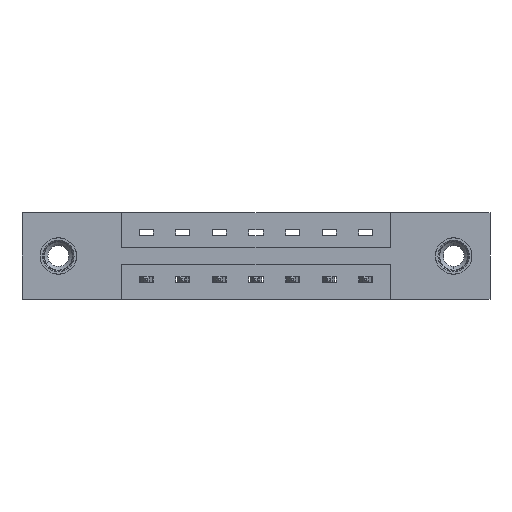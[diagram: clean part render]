
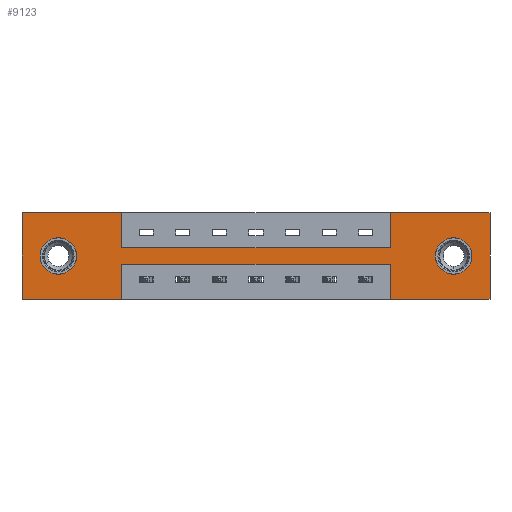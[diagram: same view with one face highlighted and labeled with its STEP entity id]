
A CAD part, front view. The second image highlights one B-rep face of the part: STEP entity #9123.
In plain terms, the highlighted planar face has unit normal (0, -1, 0).
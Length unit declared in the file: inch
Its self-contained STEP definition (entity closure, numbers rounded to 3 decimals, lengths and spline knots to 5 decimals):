
#80 = CIRCLE ( 'NONE', #4059, 0.078 ) ;
#174 = CARTESIAN_POINT ( 'NONE',  ( 1.573, 0., 0. ) ) ;
#193 = ORIENTED_EDGE ( 'NONE', *, *, #5267, .F. ) ;
#200 = DIRECTION ( 'NONE',  ( 0., 0., 1. ) ) ;
#205 = EDGE_CURVE ( 'NONE', #1161, #3313, #1393, .T. ) ;
#228 = VERTEX_POINT ( 'NONE', #9288 ) ;
#248 = DIRECTION ( 'NONE',  ( 0., 0., -1. ) ) ;
#309 = DIRECTION ( 'NONE',  ( 0., 0., -1. ) ) ;
#322 = VERTEX_POINT ( 'NONE', #9182 ) ;
#593 = EDGE_LOOP ( 'NONE', ( #8282, #1849 ) ) ;
#752 = LINE ( 'NONE', #2035, #3151 ) ;
#777 = LINE ( 'NONE', #8391, #4910 ) ;
#796 = LINE ( 'NONE', #4745, #3440 ) ;
#906 = EDGE_CURVE ( 'NONE', #228, #8220, #6104, .T. ) ;
#951 = VERTEX_POINT ( 'NONE', #7539 ) ;
#952 = CARTESIAN_POINT ( 'NONE',  ( 0.155, 0., -0.107 ) ) ;
#957 = ORIENTED_EDGE ( 'NONE', *, *, #2011, .T. ) ;
#1055 = VERTEX_POINT ( 'NONE', #5744 ) ;
#1113 = ORIENTED_EDGE ( 'NONE', *, *, #5197, .F. ) ;
#1161 = VERTEX_POINT ( 'NONE', #8983 ) ;
#1162 = DIRECTION ( 'NONE',  ( 0., 0., 1. ) ) ;
#1353 = FACE_BOUND ( 'NONE', #4217, .T. ) ;
#1393 = CIRCLE ( 'NONE', #2900, 0.078 ) ;
#1439 = CARTESIAN_POINT ( 'NONE',  ( 0.425, 0., -0.15 ) ) ;
#1481 = ORIENTED_EDGE ( 'NONE', *, *, #8433, .F. ) ;
#1596 = EDGE_LOOP ( 'NONE', ( #5784, #8561, #7151, #1766, #6206, #3369, #1481, #5132, #1113, #7271, #3338, #193 ) ) ;
#1640 = CARTESIAN_POINT ( 'NONE',  ( 0.155, 0., -0.185 ) ) ;
#1647 = VECTOR ( 'NONE', #5530, 39.37008 ) ;
#1674 = CARTESIAN_POINT ( 'NONE',  ( 0.155, 0., -0.263 ) ) ;
#1714 = EDGE_CURVE ( 'NONE', #951, #1791, #3684, .T. ) ;
#1766 = ORIENTED_EDGE ( 'NONE', *, *, #8776, .F. ) ;
#1791 = VERTEX_POINT ( 'NONE', #10866 ) ;
#1849 = ORIENTED_EDGE ( 'NONE', *, *, #7267, .T. ) ;
#2001 = VERTEX_POINT ( 'NONE', #952 ) ;
#2011 = EDGE_CURVE ( 'NONE', #10608, #2001, #5579, .T. ) ;
#2035 = CARTESIAN_POINT ( 'NONE',  ( 0., 0., 0. ) ) ;
#2158 = EDGE_CURVE ( 'NONE', #1055, #228, #3672, .T. ) ;
#2446 = CARTESIAN_POINT ( 'NONE',  ( 1.843, 0., -0.185 ) ) ;
#2522 = DIRECTION ( 'NONE',  ( -1., 0., 0. ) ) ;
#2534 = DIRECTION ( 'NONE',  ( 0., 0., 1. ) ) ;
#2651 = ORIENTED_EDGE ( 'NONE', *, *, #6670, .T. ) ;
#2759 = AXIS2_PLACEMENT_3D ( 'NONE', #10273, #5220, #1162 ) ;
#2883 = CARTESIAN_POINT ( 'NONE',  ( 0., 0., 0. ) ) ;
#2900 = AXIS2_PLACEMENT_3D ( 'NONE', #2446, #5797, #4628 ) ;
#3151 = VECTOR ( 'NONE', #200, 39.37008 ) ;
#3251 = LINE ( 'NONE', #3415, #5261 ) ;
#3313 = VERTEX_POINT ( 'NONE', #8738 ) ;
#3338 = ORIENTED_EDGE ( 'NONE', *, *, #10277, .F. ) ;
#3369 = ORIENTED_EDGE ( 'NONE', *, *, #2158, .F. ) ;
#3415 = CARTESIAN_POINT ( 'NONE',  ( 1.573, 0., -0.37 ) ) ;
#3416 = VECTOR ( 'NONE', #7264, 39.37008 ) ;
#3440 = VECTOR ( 'NONE', #309, 39.37008 ) ;
#3475 = CARTESIAN_POINT ( 'NONE',  ( 1.573, 0., -0.37 ) ) ;
#3672 = LINE ( 'NONE', #7025, #1647 ) ;
#3680 = FACE_OUTER_BOUND ( 'NONE', #1596, .T. ) ;
#3684 = LINE ( 'NONE', #2883, #3416 ) ;
#3840 = VECTOR ( 'NONE', #248, 39.37008 ) ;
#3854 = DIRECTION ( 'NONE',  ( -1., 0., 0. ) ) ;
#3856 = DIRECTION ( 'NONE',  ( 0., -1., 0. ) ) ;
#3902 = CARTESIAN_POINT ( 'NONE',  ( 1.998, 0., 0. ) ) ;
#3952 = DIRECTION ( 'NONE',  ( 0., 1., 0. ) ) ;
#4059 = AXIS2_PLACEMENT_3D ( 'NONE', #1640, #7599, #2534 ) ;
#4068 = LINE ( 'NONE', #7775, #8249 ) ;
#4153 = VERTEX_POINT ( 'NONE', #5677 ) ;
#4165 = LINE ( 'NONE', #174, #10171 ) ;
#4217 = EDGE_LOOP ( 'NONE', ( #2651, #957 ) ) ;
#4421 = EDGE_CURVE ( 'NONE', #5087, #10705, #3251, .T. ) ;
#4628 = DIRECTION ( 'NONE',  ( 0., 0., -1. ) ) ;
#4667 = CARTESIAN_POINT ( 'NONE',  ( 0.425, 0., 0. ) ) ;
#4676 = VERTEX_POINT ( 'NONE', #8818 ) ;
#4739 = CARTESIAN_POINT ( 'NONE',  ( 0., 0., -0.37 ) ) ;
#4745 = CARTESIAN_POINT ( 'NONE',  ( 0.425, 0., -0.37 ) ) ;
#4910 = VECTOR ( 'NONE', #2522, 39.37008 ) ;
#5087 = VERTEX_POINT ( 'NONE', #3475 ) ;
#5132 = ORIENTED_EDGE ( 'NONE', *, *, #10719, .F. ) ;
#5197 = EDGE_CURVE ( 'NONE', #1791, #9813, #10594, .T. ) ;
#5220 = DIRECTION ( 'NONE',  ( 0., 1., 0. ) ) ;
#5261 = VECTOR ( 'NONE', #10843, 39.37008 ) ;
#5267 = EDGE_CURVE ( 'NONE', #322, #9967, #7719, .T. ) ;
#5511 = VECTOR ( 'NONE', #3854, 39.37008 ) ;
#5514 = DIRECTION ( 'NONE',  ( 0., 0., -1. ) ) ;
#5530 = DIRECTION ( 'NONE',  ( 1., 0., 0. ) ) ;
#5579 = CIRCLE ( 'NONE', #2759, 0.078 ) ;
#5677 = CARTESIAN_POINT ( 'NONE',  ( 0.425, 0., -0.22 ) ) ;
#5744 = CARTESIAN_POINT ( 'NONE',  ( 1.573, 0., 0. ) ) ;
#5784 = ORIENTED_EDGE ( 'NONE', *, *, #7891, .F. ) ;
#5797 = DIRECTION ( 'NONE',  ( 0., 1., 0. ) ) ;
#5914 = AXIS2_PLACEMENT_3D ( 'NONE', #8937, #3952, #9744 ) ;
#5929 = CARTESIAN_POINT ( 'NONE',  ( 0., 0., -0.37 ) ) ;
#6104 = LINE ( 'NONE', #3902, #3840 ) ;
#6206 = ORIENTED_EDGE ( 'NONE', *, *, #906, .F. ) ;
#6310 = DIRECTION ( 'NONE',  ( 0., 0., 1. ) ) ;
#6670 = EDGE_CURVE ( 'NONE', #2001, #10608, #80, .T. ) ;
#7025 = CARTESIAN_POINT ( 'NONE',  ( 0., 0., 0. ) ) ;
#7151 = ORIENTED_EDGE ( 'NONE', *, *, #4421, .F. ) ;
#7264 = DIRECTION ( 'NONE',  ( 1., 0., 0. ) ) ;
#7267 = EDGE_CURVE ( 'NONE', #3313, #1161, #7561, .T. ) ;
#7271 = ORIENTED_EDGE ( 'NONE', *, *, #1714, .F. ) ;
#7539 = CARTESIAN_POINT ( 'NONE',  ( 0., 0., 0. ) ) ;
#7561 = CIRCLE ( 'NONE', #5914, 0.078 ) ;
#7599 = DIRECTION ( 'NONE',  ( 0., 1., 0. ) ) ;
#7719 = LINE ( 'NONE', #4739, #5511 ) ;
#7735 = CARTESIAN_POINT ( 'NONE',  ( 1.573, 0., -0.22 ) ) ;
#7775 = CARTESIAN_POINT ( 'NONE',  ( 0.425, 0., -0.15 ) ) ;
#7836 = EDGE_CURVE ( 'NONE', #10705, #4153, #10557, .T. ) ;
#7891 = EDGE_CURVE ( 'NONE', #4153, #322, #796, .T. ) ;
#7900 = FACE_BOUND ( 'NONE', #593, .T. ) ;
#7965 = VECTOR ( 'NONE', #5514, 39.37008 ) ;
#7976 = DIRECTION ( 'NONE',  ( -1., 0., 0. ) ) ;
#8000 = AXIS2_PLACEMENT_3D ( 'NONE', #8842, #3856, #9660 ) ;
#8174 = VECTOR ( 'NONE', #7976, 39.37008 ) ;
#8220 = VERTEX_POINT ( 'NONE', #10078 ) ;
#8249 = VECTOR ( 'NONE', #8562, 39.37008 ) ;
#8282 = ORIENTED_EDGE ( 'NONE', *, *, #205, .T. ) ;
#8391 = CARTESIAN_POINT ( 'NONE',  ( 0., 0., -0.37 ) ) ;
#8433 = EDGE_CURVE ( 'NONE', #4676, #1055, #4165, .T. ) ;
#8561 = ORIENTED_EDGE ( 'NONE', *, *, #7836, .F. ) ;
#8562 = DIRECTION ( 'NONE',  ( 1., 0., 0. ) ) ;
#8738 = CARTESIAN_POINT ( 'NONE',  ( 1.843, 0., -0.263 ) ) ;
#8776 = EDGE_CURVE ( 'NONE', #8220, #5087, #777, .T. ) ;
#8818 = CARTESIAN_POINT ( 'NONE',  ( 1.573, 0., -0.15 ) ) ;
#8842 = CARTESIAN_POINT ( 'NONE',  ( 0., 0., -0.37 ) ) ;
#8937 = CARTESIAN_POINT ( 'NONE',  ( 1.843, 0., -0.185 ) ) ;
#8983 = CARTESIAN_POINT ( 'NONE',  ( 1.843, 0., -0.107 ) ) ;
#9123 = ADVANCED_FACE ( 'NONE', ( #7900, #1353, #3680 ), #10425, .T. ) ;
#9182 = CARTESIAN_POINT ( 'NONE',  ( 0.425, 0., -0.37 ) ) ;
#9288 = CARTESIAN_POINT ( 'NONE',  ( 1.998, 0., 0. ) ) ;
#9660 = DIRECTION ( 'NONE',  ( 0., 0., -1. ) ) ;
#9744 = DIRECTION ( 'NONE',  ( 0., 0., -1. ) ) ;
#9813 = VERTEX_POINT ( 'NONE', #1439 ) ;
#9967 = VERTEX_POINT ( 'NONE', #5929 ) ;
#10078 = CARTESIAN_POINT ( 'NONE',  ( 1.998, 0., -0.37 ) ) ;
#10171 = VECTOR ( 'NONE', #6310, 39.37008 ) ;
#10273 = CARTESIAN_POINT ( 'NONE',  ( 0.155, 0., -0.185 ) ) ;
#10277 = EDGE_CURVE ( 'NONE', #9967, #951, #752, .T. ) ;
#10356 = CARTESIAN_POINT ( 'NONE',  ( 0.425, 0., -0.22 ) ) ;
#10425 = PLANE ( 'NONE',  #8000 ) ;
#10557 = LINE ( 'NONE', #10356, #8174 ) ;
#10594 = LINE ( 'NONE', #4667, #7965 ) ;
#10608 = VERTEX_POINT ( 'NONE', #1674 ) ;
#10705 = VERTEX_POINT ( 'NONE', #7735 ) ;
#10719 = EDGE_CURVE ( 'NONE', #9813, #4676, #4068, .T. ) ;
#10843 = DIRECTION ( 'NONE',  ( 0., 0., 1. ) ) ;
#10866 = CARTESIAN_POINT ( 'NONE',  ( 0.425, 0., 0. ) ) ;
